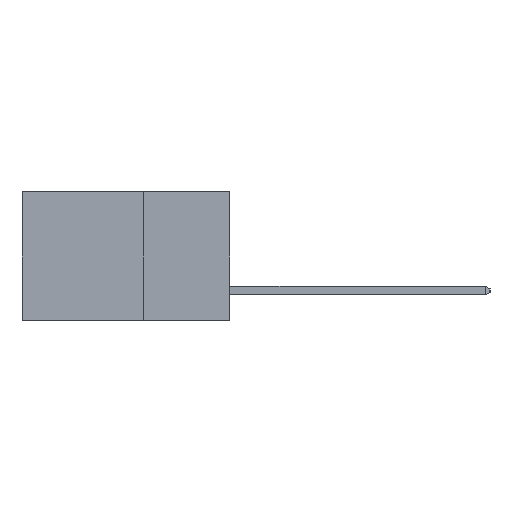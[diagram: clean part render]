
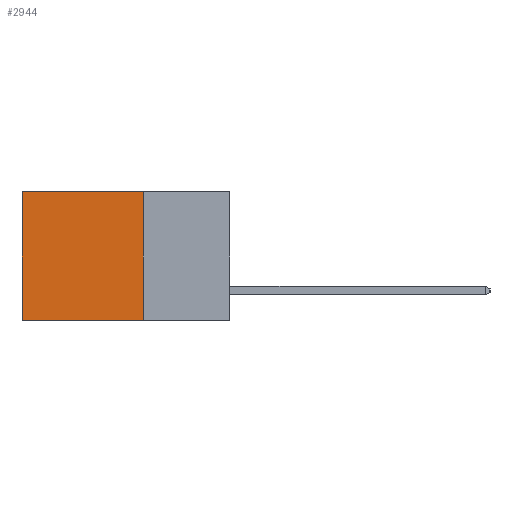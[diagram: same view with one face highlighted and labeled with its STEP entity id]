
A CAD part, left-side view. The second image highlights one B-rep face of the part: STEP entity #2944.
In plain terms, the highlighted planar face has unit normal (-1, 0, 0).
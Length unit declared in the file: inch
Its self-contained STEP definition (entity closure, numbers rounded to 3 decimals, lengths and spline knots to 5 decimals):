
#1202 = LINE ( 'NONE', #3355, #11146 ) ;
#1364 = DIRECTION ( 'NONE',  ( 0., 1., 0. ) ) ;
#1715 = VECTOR ( 'NONE', #1364, 39.37008 ) ;
#2942 = LINE ( 'NONE', #12401, #7001 ) ;
#2944 = ADVANCED_FACE ( 'NONE', ( #20437 ), #22138, .F. ) ;
#3355 = CARTESIAN_POINT ( 'NONE',  ( 0.2615, 0.6, -0.37 ) ) ;
#4519 = EDGE_CURVE ( 'NONE', #7617, #21441, #2942, .T. ) ;
#6186 = ORIENTED_EDGE ( 'NONE', *, *, #12764, .F. ) ;
#6415 = LINE ( 'NONE', #13233, #1715 ) ;
#7001 = VECTOR ( 'NONE', #17247, 39.37008 ) ;
#7617 = VERTEX_POINT ( 'NONE', #18794 ) ;
#7620 = VECTOR ( 'NONE', #13980, 39.37008 ) ;
#8034 = CARTESIAN_POINT ( 'NONE',  ( 0.2615, 0.25, -0.37 ) ) ;
#10542 = ORIENTED_EDGE ( 'NONE', *, *, #20909, .T. ) ;
#10821 = AXIS2_PLACEMENT_3D ( 'NONE', #24312, #21629, #14141 ) ;
#11146 = VECTOR ( 'NONE', #19208, 39.37008 ) ;
#12401 = CARTESIAN_POINT ( 'NONE',  ( 0.2615, 0.25, -0.37 ) ) ;
#12764 = EDGE_CURVE ( 'NONE', #18982, #7617, #23272, .T. ) ;
#13073 = VERTEX_POINT ( 'NONE', #14812 ) ;
#13233 = CARTESIAN_POINT ( 'NONE',  ( 0.2615, 0.25, 0. ) ) ;
#13980 = DIRECTION ( 'NONE',  ( 0., 0., -1. ) ) ;
#14141 = DIRECTION ( 'NONE',  ( 0., 0., -1. ) ) ;
#14812 = CARTESIAN_POINT ( 'NONE',  ( 0.2615, 0.6, 0. ) ) ;
#16132 = CARTESIAN_POINT ( 'NONE',  ( 0.2615, 0.6, -0.37 ) ) ;
#16616 = EDGE_CURVE ( 'NONE', #18982, #13073, #6415, .T. ) ;
#17247 = DIRECTION ( 'NONE',  ( 0., 1., 0. ) ) ;
#17957 = EDGE_LOOP ( 'NONE', ( #10542, #21132, #6186, #25069 ) ) ;
#18794 = CARTESIAN_POINT ( 'NONE',  ( 0.2615, 0.25, -0.37 ) ) ;
#18982 = VERTEX_POINT ( 'NONE', #25007 ) ;
#19208 = DIRECTION ( 'NONE',  ( 0., 0., -1. ) ) ;
#20437 = FACE_OUTER_BOUND ( 'NONE', #17957, .T. ) ;
#20909 = EDGE_CURVE ( 'NONE', #13073, #21441, #1202, .T. ) ;
#21132 = ORIENTED_EDGE ( 'NONE', *, *, #4519, .F. ) ;
#21441 = VERTEX_POINT ( 'NONE', #16132 ) ;
#21629 = DIRECTION ( 'NONE',  ( 1., 0., 0. ) ) ;
#22138 = PLANE ( 'NONE',  #10821 ) ;
#23272 = LINE ( 'NONE', #8034, #7620 ) ;
#24312 = CARTESIAN_POINT ( 'NONE',  ( 0.2615, 0.25, -0.37 ) ) ;
#25007 = CARTESIAN_POINT ( 'NONE',  ( 0.2615, 0.25, 0. ) ) ;
#25069 = ORIENTED_EDGE ( 'NONE', *, *, #16616, .T. ) ;
